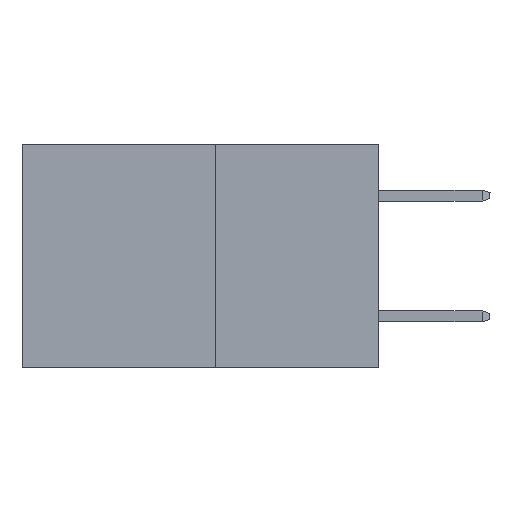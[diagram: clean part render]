
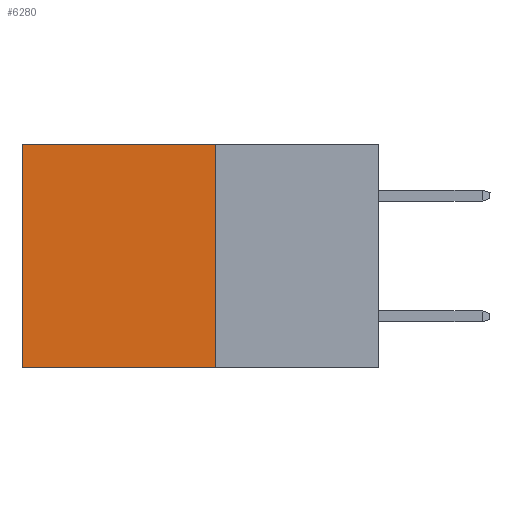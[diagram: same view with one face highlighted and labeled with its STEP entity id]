
A CAD part, left-side view. The second image highlights one B-rep face of the part: STEP entity #6280.
In plain terms, the highlighted planar face has unit normal (-1, 0, 0).
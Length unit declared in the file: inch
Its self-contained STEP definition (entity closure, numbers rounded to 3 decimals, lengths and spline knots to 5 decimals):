
#577 = CARTESIAN_POINT ( 'NONE',  ( 0.277, 0.27, -0.37 ) ) ;
#585 = VERTEX_POINT ( 'NONE', #2212 ) ;
#1152 = CARTESIAN_POINT ( 'NONE',  ( 0.277, 0.27, 0. ) ) ;
#1657 = EDGE_CURVE ( 'NONE', #13635, #4329, #5328, .T. ) ;
#2212 = CARTESIAN_POINT ( 'NONE',  ( 0.277, 0.27, -0.37 ) ) ;
#2734 = DIRECTION ( 'NONE',  ( 0., 1., 0. ) ) ;
#3094 = LINE ( 'NONE', #1152, #10642 ) ;
#3216 = ORIENTED_EDGE ( 'NONE', *, *, #1657, .T. ) ;
#3473 = CARTESIAN_POINT ( 'NONE',  ( 0.277, 0.59, -0.37 ) ) ;
#3793 = EDGE_CURVE ( 'NONE', #3880, #585, #16092, .T. ) ;
#3852 = EDGE_CURVE ( 'NONE', #585, #4329, #15658, .T. ) ;
#3880 = VERTEX_POINT ( 'NONE', #13432 ) ;
#4244 = EDGE_LOOP ( 'NONE', ( #3216, #7188, #11228, #7675 ) ) ;
#4329 = VERTEX_POINT ( 'NONE', #3473 ) ;
#5328 = LINE ( 'NONE', #12814, #9307 ) ;
#6280 = ADVANCED_FACE ( 'NONE', ( #18907 ), #17515, .F. ) ;
#7188 = ORIENTED_EDGE ( 'NONE', *, *, #3852, .F. ) ;
#7211 = VECTOR ( 'NONE', #9220, 39.37008 ) ;
#7295 = CARTESIAN_POINT ( 'NONE',  ( 0.277, 0.59, 0. ) ) ;
#7675 = ORIENTED_EDGE ( 'NONE', *, *, #16753, .T. ) ;
#7990 = AXIS2_PLACEMENT_3D ( 'NONE', #17462, #17447, #17445 ) ;
#9154 = DIRECTION ( 'NONE',  ( 0., 0., -1. ) ) ;
#9220 = DIRECTION ( 'NONE',  ( 0., 1., 0. ) ) ;
#9307 = VECTOR ( 'NONE', #9154, 39.37008 ) ;
#10617 = DIRECTION ( 'NONE',  ( 0., 0., -1. ) ) ;
#10642 = VECTOR ( 'NONE', #2734, 39.37008 ) ;
#11228 = ORIENTED_EDGE ( 'NONE', *, *, #3793, .F. ) ;
#12220 = VECTOR ( 'NONE', #10617, 39.37008 ) ;
#12814 = CARTESIAN_POINT ( 'NONE',  ( 0.277, 0.59, -0.37 ) ) ;
#13432 = CARTESIAN_POINT ( 'NONE',  ( 0.277, 0.27, 0. ) ) ;
#13513 = CARTESIAN_POINT ( 'NONE',  ( 0.277, 0.27, -0.37 ) ) ;
#13635 = VERTEX_POINT ( 'NONE', #7295 ) ;
#15658 = LINE ( 'NONE', #577, #7211 ) ;
#16092 = LINE ( 'NONE', #13513, #12220 ) ;
#16753 = EDGE_CURVE ( 'NONE', #3880, #13635, #3094, .T. ) ;
#17445 = DIRECTION ( 'NONE',  ( 0., 0., -1. ) ) ;
#17447 = DIRECTION ( 'NONE',  ( 1., 0., 0. ) ) ;
#17462 = CARTESIAN_POINT ( 'NONE',  ( 0.277, 0.27, -0.37 ) ) ;
#17515 = PLANE ( 'NONE',  #7990 ) ;
#18907 = FACE_OUTER_BOUND ( 'NONE', #4244, .T. ) ;
